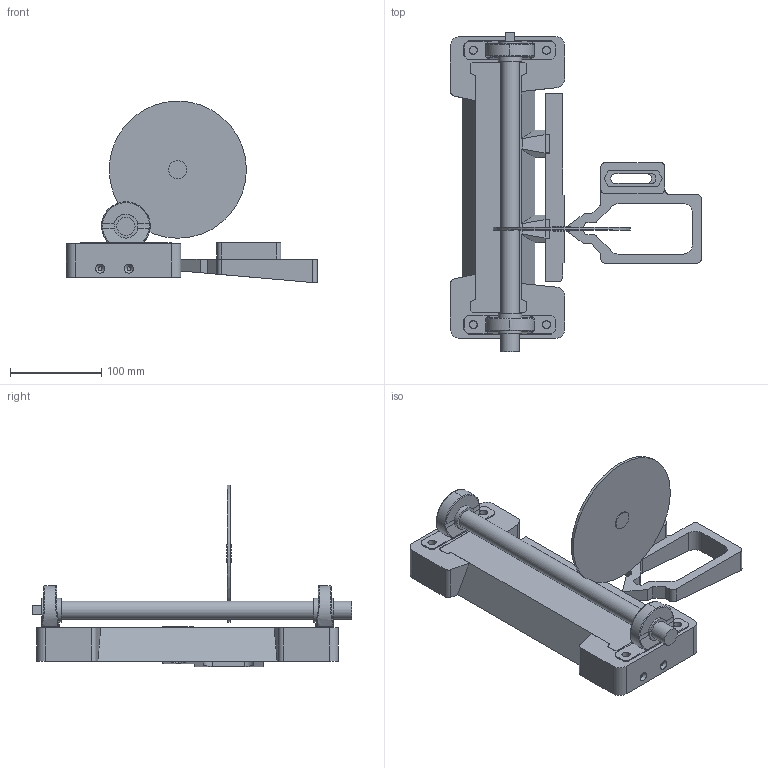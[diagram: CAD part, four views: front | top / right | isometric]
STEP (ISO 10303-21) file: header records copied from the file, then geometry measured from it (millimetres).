
FILE_DESCRIPTION(/* description */ (''),/* implementation_level */ '2;1');
FILE_NAME(/* author */ (''),/* organization */ (''),/* preprocessor_version */ 'ST-DEVELOPER v15.2',/* originating_system */ 'Autodesk Translator Framework v2.0.0.5431',/* authorisation */ '');
FILE_SCHEMA (('AUTOMOTIVE_DESIGN { 1 0 10303 214 3 1 1 }'));
Length unit declared in the file: centimetre
Products named in the file (1): HOMEMADE BOLT LATHE V6
Bounding box: 274.5 x 349 x 198.86 mm (x, y, z)
Volume: 1324664 mm3; surface area: 289577.8 mm2
Topology: 10 solids, 10 shells, 356 faces, 918 edges, 593 vertices
Faces by surface type: plane 225, cylinder 85, bspline 28, cone 18
Full cylindrical faces by diameter (mm): 4 x12, 8.4 x4, 9 x4, 20 x5, 26 x4, 150 x1
Entity records: 11631 total; most frequent: CARTESIAN_POINT 3184, ORIENTED_EDGE 1708, DIRECTION 1638, EDGE_CURVE 854, LINE 588, VECTOR 588, VERTEX_POINT 585, AXIS2_PLACEMENT_3D 525
